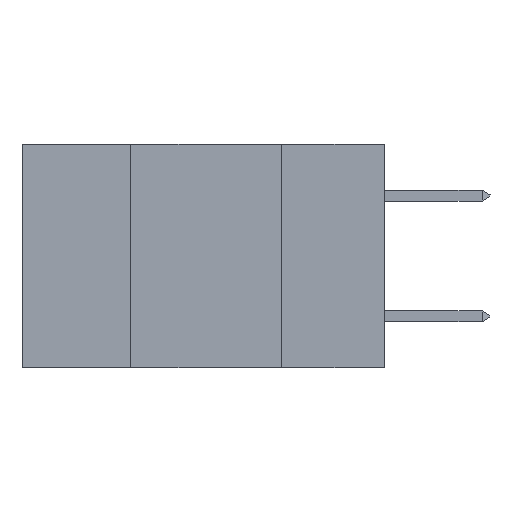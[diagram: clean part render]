
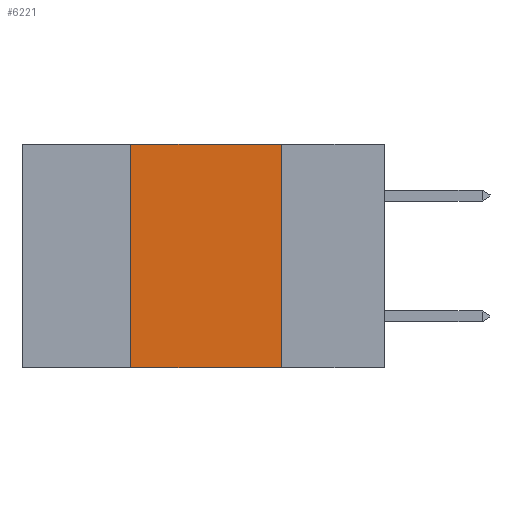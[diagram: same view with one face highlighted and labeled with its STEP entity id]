
A CAD part, left-side view. The second image highlights one B-rep face of the part: STEP entity #6221.
In plain terms, the highlighted planar face has unit normal (-1, 0, 0).
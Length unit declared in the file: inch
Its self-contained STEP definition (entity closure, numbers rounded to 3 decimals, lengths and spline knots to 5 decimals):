
#251 = VECTOR ( 'NONE', #1191, 39.37008 ) ;
#352 = CARTESIAN_POINT ( 'NONE',  ( 0., 0.42, -0.37 ) ) ;
#557 = DIRECTION ( 'NONE',  ( 0., -1., 0. ) ) ;
#1059 = CARTESIAN_POINT ( 'NONE',  ( 0., 0.42, 0. ) ) ;
#1191 = DIRECTION ( 'NONE',  ( 0., 0., 1. ) ) ;
#1748 = VERTEX_POINT ( 'NONE', #29097 ) ;
#2568 = CARTESIAN_POINT ( 'NONE',  ( 0., 0.17, 0. ) ) ;
#3286 = LINE ( 'NONE', #15131, #251 ) ;
#6221 = ADVANCED_FACE ( 'NONE', ( #16766 ), #7238, .F. ) ;
#7238 = PLANE ( 'NONE',  #7322 ) ;
#7322 = AXIS2_PLACEMENT_3D ( 'NONE', #23588, #12301, #18082 ) ;
#7923 = EDGE_CURVE ( 'NONE', #14958, #16797, #3286, .T. ) ;
#10452 = VECTOR ( 'NONE', #32026, 39.37008 ) ;
#11119 = CARTESIAN_POINT ( 'NONE',  ( 0., 0.17, 0. ) ) ;
#11420 = EDGE_CURVE ( 'NONE', #16797, #26388, #25072, .T. ) ;
#12301 = DIRECTION ( 'NONE',  ( 1., 0., 0. ) ) ;
#12304 = CARTESIAN_POINT ( 'NONE',  ( 0., 0.6, 0. ) ) ;
#14958 = VERTEX_POINT ( 'NONE', #352 ) ;
#15102 = CARTESIAN_POINT ( 'NONE',  ( 0., 0.6, -0.37 ) ) ;
#15131 = CARTESIAN_POINT ( 'NONE',  ( 0., 0.42, 0. ) ) ;
#15448 = EDGE_CURVE ( 'NONE', #14958, #1748, #16097, .T. ) ;
#16097 = LINE ( 'NONE', #15102, #26432 ) ;
#16766 = FACE_OUTER_BOUND ( 'NONE', #21676, .T. ) ;
#16797 = VERTEX_POINT ( 'NONE', #1059 ) ;
#18082 = DIRECTION ( 'NONE',  ( 0., 0., -1. ) ) ;
#20935 = ORIENTED_EDGE ( 'NONE', *, *, #11420, .F. ) ;
#21676 = EDGE_LOOP ( 'NONE', ( #28473, #20935, #23245, #29641 ) ) ;
#22253 = EDGE_CURVE ( 'NONE', #26388, #1748, #29478, .T. ) ;
#23245 = ORIENTED_EDGE ( 'NONE', *, *, #7923, .F. ) ;
#23588 = CARTESIAN_POINT ( 'NONE',  ( 0., 0.6, 0. ) ) ;
#25072 = LINE ( 'NONE', #12304, #10452 ) ;
#25158 = DIRECTION ( 'NONE',  ( 0., 0., -1. ) ) ;
#26388 = VERTEX_POINT ( 'NONE', #11119 ) ;
#26432 = VECTOR ( 'NONE', #557, 39.37008 ) ;
#27435 = VECTOR ( 'NONE', #25158, 39.37008 ) ;
#28473 = ORIENTED_EDGE ( 'NONE', *, *, #22253, .F. ) ;
#29097 = CARTESIAN_POINT ( 'NONE',  ( 0., 0.17, -0.37 ) ) ;
#29478 = LINE ( 'NONE', #2568, #27435 ) ;
#29641 = ORIENTED_EDGE ( 'NONE', *, *, #15448, .T. ) ;
#32026 = DIRECTION ( 'NONE',  ( 0., -1., 0. ) ) ;
